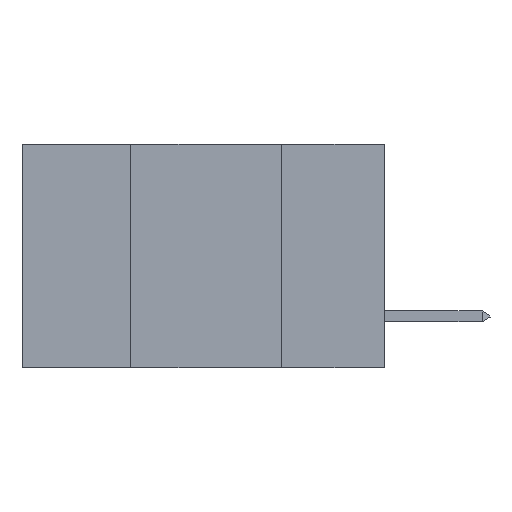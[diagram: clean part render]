
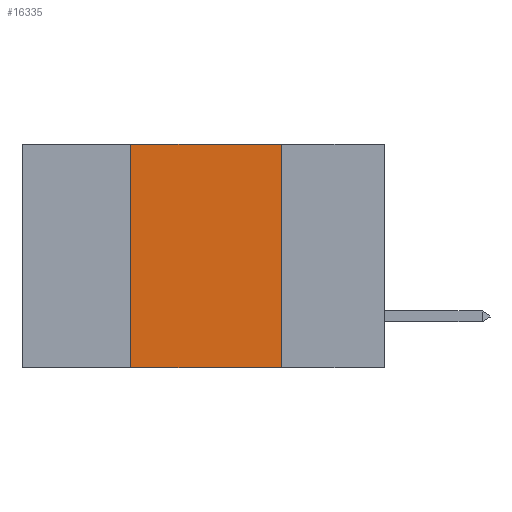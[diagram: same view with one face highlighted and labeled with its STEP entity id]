
A CAD part, left-side view. The second image highlights one B-rep face of the part: STEP entity #16335.
In plain terms, the highlighted planar face has unit normal (-1, 0, 0).
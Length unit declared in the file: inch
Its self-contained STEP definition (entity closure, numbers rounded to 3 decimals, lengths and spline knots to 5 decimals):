
#1286 = LINE ( 'NONE', #7809, #44109 ) ;
#3307 = DIRECTION ( 'NONE',  ( 0., 0., -1. ) ) ;
#3760 = LINE ( 'NONE', #25694, #32346 ) ;
#3803 = ORIENTED_EDGE ( 'NONE', *, *, #17321, .F. ) ;
#6215 = DIRECTION ( 'NONE',  ( 0., -1., 0. ) ) ;
#6716 = CARTESIAN_POINT ( 'NONE',  ( 0., 0.6, 0. ) ) ;
#7618 = CARTESIAN_POINT ( 'NONE',  ( 0., 0.17, 0. ) ) ;
#7809 = CARTESIAN_POINT ( 'NONE',  ( 0., 0.42, 0. ) ) ;
#8398 = DIRECTION ( 'NONE',  ( 0., -1., 0. ) ) ;
#10602 = ORIENTED_EDGE ( 'NONE', *, *, #26420, .F. ) ;
#10708 = CARTESIAN_POINT ( 'NONE',  ( 0., 0.42, -0.37 ) ) ;
#15287 = PLANE ( 'NONE',  #21904 ) ;
#16335 = ADVANCED_FACE ( 'NONE', ( #45918 ), #15287, .F. ) ;
#16831 = EDGE_CURVE ( 'NONE', #27658, #22438, #3760, .T. ) ;
#17321 = EDGE_CURVE ( 'NONE', #20394, #40811, #1286, .T. ) ;
#18738 = CARTESIAN_POINT ( 'NONE',  ( 0., 0.6, 0. ) ) ;
#20394 = VERTEX_POINT ( 'NONE', #10708 ) ;
#21904 = AXIS2_PLACEMENT_3D ( 'NONE', #18738, #41473, #41637 ) ;
#22438 = VERTEX_POINT ( 'NONE', #26611 ) ;
#22538 = ORIENTED_EDGE ( 'NONE', *, *, #16831, .F. ) ;
#23836 = DIRECTION ( 'NONE',  ( 0., 0., 1. ) ) ;
#25694 = CARTESIAN_POINT ( 'NONE',  ( 0., 0.17, 0. ) ) ;
#26420 = EDGE_CURVE ( 'NONE', #40811, #27658, #26491, .T. ) ;
#26491 = LINE ( 'NONE', #6716, #44730 ) ;
#26611 = CARTESIAN_POINT ( 'NONE',  ( 0., 0.17, -0.37 ) ) ;
#27658 = VERTEX_POINT ( 'NONE', #7618 ) ;
#29132 = EDGE_CURVE ( 'NONE', #20394, #22438, #30688, .T. ) ;
#30688 = LINE ( 'NONE', #32150, #37163 ) ;
#32074 = ORIENTED_EDGE ( 'NONE', *, *, #29132, .T. ) ;
#32150 = CARTESIAN_POINT ( 'NONE',  ( 0., 0.6, -0.37 ) ) ;
#32346 = VECTOR ( 'NONE', #3307, 39.37008 ) ;
#33592 = EDGE_LOOP ( 'NONE', ( #22538, #10602, #3803, #32074 ) ) ;
#37163 = VECTOR ( 'NONE', #6215, 39.37008 ) ;
#40811 = VERTEX_POINT ( 'NONE', #42317 ) ;
#41473 = DIRECTION ( 'NONE',  ( 1., 0., 0. ) ) ;
#41637 = DIRECTION ( 'NONE',  ( 0., 0., -1. ) ) ;
#42317 = CARTESIAN_POINT ( 'NONE',  ( 0., 0.42, 0. ) ) ;
#44109 = VECTOR ( 'NONE', #23836, 39.37008 ) ;
#44730 = VECTOR ( 'NONE', #8398, 39.37008 ) ;
#45918 = FACE_OUTER_BOUND ( 'NONE', #33592, .T. ) ;
